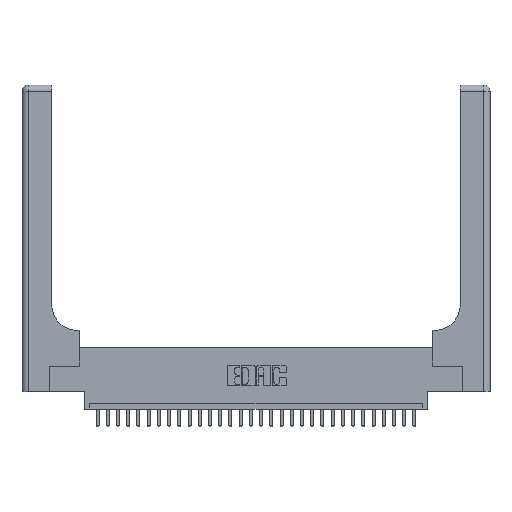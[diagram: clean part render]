
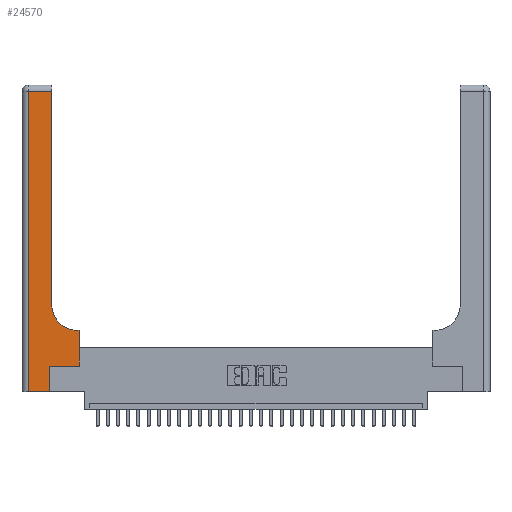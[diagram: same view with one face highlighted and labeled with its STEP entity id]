
A CAD part, top view. The second image highlights one B-rep face of the part: STEP entity #24570.
In plain terms, the highlighted planar face has unit normal (0, 0, 1).
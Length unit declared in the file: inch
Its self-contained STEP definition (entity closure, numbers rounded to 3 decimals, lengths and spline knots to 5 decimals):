
#308 = CARTESIAN_POINT ( 'NONE',  ( 0.269, 0.25, 0.37 ) ) ;
#387 = CARTESIAN_POINT ( 'NONE',  ( 0.2915, 0.85, 0.37 ) ) ;
#1036 = AXIS2_PLACEMENT_3D ( 'NONE', #28181, #13877, #1809 ) ;
#1675 = VERTEX_POINT ( 'NONE', #25788 ) ;
#1809 = DIRECTION ( 'NONE',  ( 1., 0., 0. ) ) ;
#2265 = CARTESIAN_POINT ( 'NONE',  ( 0., 3., 0.37 ) ) ;
#2800 = ORIENTED_EDGE ( 'NONE', *, *, #16141, .T. ) ;
#3347 = ORIENTED_EDGE ( 'NONE', *, *, #9206, .T. ) ;
#3881 = VECTOR ( 'NONE', #20267, 39.37008 ) ;
#5070 = CARTESIAN_POINT ( 'NONE',  ( 0.2915, 0.6, 0.37 ) ) ;
#5936 = LINE ( 'NONE', #25134, #8544 ) ;
#5971 = EDGE_CURVE ( 'NONE', #30352, #20359, #12816, .T. ) ;
#6049 = DIRECTION ( 'NONE',  ( 0., -1., 0. ) ) ;
#6906 = FACE_OUTER_BOUND ( 'NONE', #7696, .T. ) ;
#7216 = VERTEX_POINT ( 'NONE', #11055 ) ;
#7696 = EDGE_LOOP ( 'NONE', ( #22397, #2800, #19818, #28314, #3347, #9287, #27433, #19632, #14306 ) ) ;
#7923 = VERTEX_POINT ( 'NONE', #26628 ) ;
#7965 = LINE ( 'NONE', #8853, #17246 ) ;
#8544 = VECTOR ( 'NONE', #20151, 39.37008 ) ;
#8853 = CARTESIAN_POINT ( 'NONE',  ( 0.2915, 3., 0.37 ) ) ;
#9145 = CARTESIAN_POINT ( 'NONE',  ( 0.269, 0., 0.37 ) ) ;
#9206 = EDGE_CURVE ( 'NONE', #1675, #30352, #20134, .T. ) ;
#9287 = ORIENTED_EDGE ( 'NONE', *, *, #5971, .T. ) ;
#9289 = CARTESIAN_POINT ( 'NONE',  ( 0.5415, 0.6, 0.37 ) ) ;
#9700 = CARTESIAN_POINT ( 'NONE',  ( 0.06, 0., 0.37 ) ) ;
#9773 = EDGE_CURVE ( 'NONE', #7216, #25299, #19382, .T. ) ;
#10941 = CARTESIAN_POINT ( 'NONE',  ( 0., 0., 0.37 ) ) ;
#11055 = CARTESIAN_POINT ( 'NONE',  ( 0.5585, 0.6, 0.37 ) ) ;
#11881 = EDGE_CURVE ( 'NONE', #25299, #17446, #12536, .T. ) ;
#12536 = CIRCLE ( 'NONE', #1036, 0.25 ) ;
#12816 = LINE ( 'NONE', #308, #17233 ) ;
#13353 = DIRECTION ( 'NONE',  ( 1., 0., 0. ) ) ;
#13782 = VECTOR ( 'NONE', #30213, 39.37008 ) ;
#13817 = DIRECTION ( 'NONE',  ( -1., 0., 0. ) ) ;
#13877 = DIRECTION ( 'NONE',  ( 0., 0., -1. ) ) ;
#14130 = DIRECTION ( 'NONE',  ( 1., 0., 0. ) ) ;
#14306 = ORIENTED_EDGE ( 'NONE', *, *, #11881, .T. ) ;
#14529 = VECTOR ( 'NONE', #19470, 39.37008 ) ;
#14614 = EDGE_CURVE ( 'NONE', #29035, #1675, #18693, .T. ) ;
#16141 = EDGE_CURVE ( 'NONE', #18922, #7923, #5936, .T. ) ;
#16529 = LINE ( 'NONE', #29856, #3881 ) ;
#17233 = VECTOR ( 'NONE', #14130, 39.37008 ) ;
#17246 = VECTOR ( 'NONE', #27734, 39.37008 ) ;
#17446 = VERTEX_POINT ( 'NONE', #387 ) ;
#18484 = DIRECTION ( 'NONE',  ( 0., 0., -1. ) ) ;
#18693 = LINE ( 'NONE', #10941, #21349 ) ;
#18767 = VECTOR ( 'NONE', #6049, 39.37008 ) ;
#18922 = VERTEX_POINT ( 'NONE', #27381 ) ;
#19382 = LINE ( 'NONE', #5070, #14529 ) ;
#19470 = DIRECTION ( 'NONE',  ( -1., 0., 0. ) ) ;
#19632 = ORIENTED_EDGE ( 'NONE', *, *, #9773, .T. ) ;
#19672 = EDGE_CURVE ( 'NONE', #20359, #7216, #16529, .T. ) ;
#19805 = LINE ( 'NONE', #27220, #18767 ) ;
#19818 = ORIENTED_EDGE ( 'NONE', *, *, #22601, .T. ) ;
#20134 = LINE ( 'NONE', #9145, #13782 ) ;
#20151 = DIRECTION ( 'NONE',  ( -1., 0., 0. ) ) ;
#20267 = DIRECTION ( 'NONE',  ( 0., 1., 0. ) ) ;
#20359 = VERTEX_POINT ( 'NONE', #22927 ) ;
#21349 = VECTOR ( 'NONE', #13353, 39.37008 ) ;
#22397 = ORIENTED_EDGE ( 'NONE', *, *, #25607, .T. ) ;
#22601 = EDGE_CURVE ( 'NONE', #7923, #29035, #19805, .T. ) ;
#22927 = CARTESIAN_POINT ( 'NONE',  ( 0.5585, 0.25, 0.37 ) ) ;
#23107 = PLANE ( 'NONE',  #28591 ) ;
#24570 = ADVANCED_FACE ( 'NONE', ( #6906 ), #23107, .F. ) ;
#25134 = CARTESIAN_POINT ( 'NONE',  ( 0., 2.94, 0.37 ) ) ;
#25299 = VERTEX_POINT ( 'NONE', #9289 ) ;
#25352 = CARTESIAN_POINT ( 'NONE',  ( 0.269, 0.25, 0.37 ) ) ;
#25607 = EDGE_CURVE ( 'NONE', #17446, #18922, #7965, .T. ) ;
#25788 = CARTESIAN_POINT ( 'NONE',  ( 0.269, 0., 0.37 ) ) ;
#26628 = CARTESIAN_POINT ( 'NONE',  ( 0.06, 2.94, 0.37 ) ) ;
#27220 = CARTESIAN_POINT ( 'NONE',  ( 0.06, 3., 0.37 ) ) ;
#27381 = CARTESIAN_POINT ( 'NONE',  ( 0.2915, 2.94, 0.37 ) ) ;
#27433 = ORIENTED_EDGE ( 'NONE', *, *, #19672, .T. ) ;
#27734 = DIRECTION ( 'NONE',  ( 0., 1., 0. ) ) ;
#28181 = CARTESIAN_POINT ( 'NONE',  ( 0.5415, 0.85, 0.37 ) ) ;
#28314 = ORIENTED_EDGE ( 'NONE', *, *, #14614, .T. ) ;
#28591 = AXIS2_PLACEMENT_3D ( 'NONE', #2265, #18484, #13817 ) ;
#29035 = VERTEX_POINT ( 'NONE', #9700 ) ;
#29856 = CARTESIAN_POINT ( 'NONE',  ( 0.5585, 0.25, 0.37 ) ) ;
#30213 = DIRECTION ( 'NONE',  ( 0., 1., 0. ) ) ;
#30352 = VERTEX_POINT ( 'NONE', #25352 ) ;
